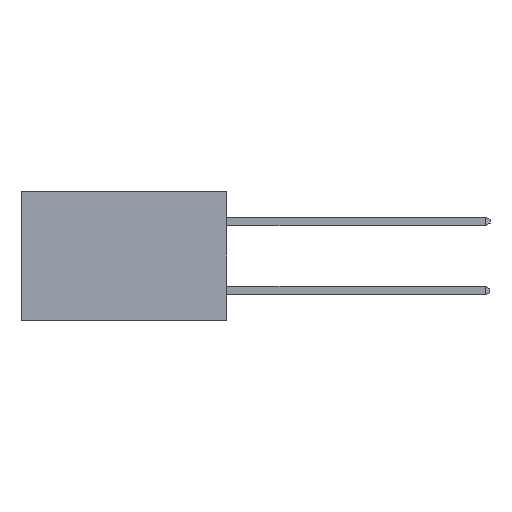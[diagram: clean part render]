
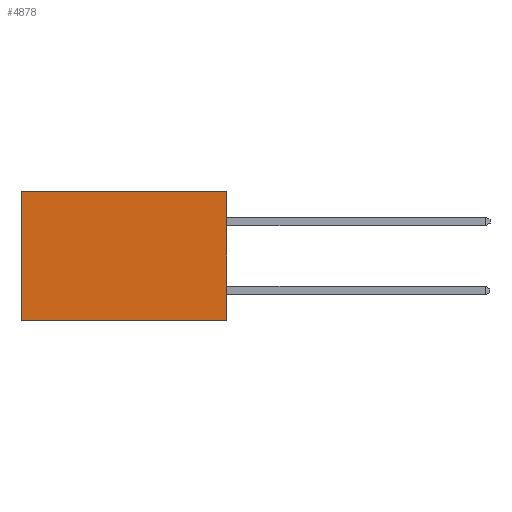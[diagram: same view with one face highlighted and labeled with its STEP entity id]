
A CAD part, left-side view. The second image highlights one B-rep face of the part: STEP entity #4878.
In plain terms, the highlighted planar face has unit normal (-1, 0, 0).
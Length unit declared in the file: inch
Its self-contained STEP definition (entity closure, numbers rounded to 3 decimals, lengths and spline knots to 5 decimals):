
#262 = VERTEX_POINT ( 'NONE', #10888 ) ;
#295 = ORIENTED_EDGE ( 'NONE', *, *, #1447, .F. ) ;
#546 = ORIENTED_EDGE ( 'NONE', *, *, #5599, .F. ) ;
#655 = ORIENTED_EDGE ( 'NONE', *, *, #930, .T. ) ;
#930 = EDGE_CURVE ( 'NONE', #1466, #262, #5313, .T. ) ;
#1001 = LINE ( 'NONE', #2396, #2843 ) ;
#1375 = EDGE_CURVE ( 'NONE', #262, #5024, #5073, .T. ) ;
#1444 = ORIENTED_EDGE ( 'NONE', *, *, #1375, .T. ) ;
#1447 = EDGE_CURVE ( 'NONE', #11264, #5024, #10744, .T. ) ;
#1466 = VERTEX_POINT ( 'NONE', #10134 ) ;
#2111 = DIRECTION ( 'NONE',  ( 0., 1., 0. ) ) ;
#2130 = AXIS2_PLACEMENT_3D ( 'NONE', #4250, #5791, #5788 ) ;
#2308 = DIRECTION ( 'NONE',  ( 0., 0., -1. ) ) ;
#2396 = CARTESIAN_POINT ( 'NONE',  ( 0.277, 0., -0.37 ) ) ;
#2786 = VECTOR ( 'NONE', #10671, 39.37008 ) ;
#2843 = VECTOR ( 'NONE', #2308, 39.37008 ) ;
#3732 = VECTOR ( 'NONE', #2111, 39.37008 ) ;
#4171 = DIRECTION ( 'NONE',  ( 0., 0., -1. ) ) ;
#4250 = CARTESIAN_POINT ( 'NONE',  ( 0.277, 0., -0.37 ) ) ;
#4266 = PLANE ( 'NONE',  #2130 ) ;
#4386 = CARTESIAN_POINT ( 'NONE',  ( 0.277, 0.59, -0.37 ) ) ;
#4878 = ADVANCED_FACE ( 'NONE', ( #5660 ), #4266, .F. ) ;
#5024 = VERTEX_POINT ( 'NONE', #4386 ) ;
#5073 = LINE ( 'NONE', #5086, #7160 ) ;
#5086 = CARTESIAN_POINT ( 'NONE',  ( 0.277, 0.59, -0.37 ) ) ;
#5313 = LINE ( 'NONE', #10968, #2786 ) ;
#5599 = EDGE_CURVE ( 'NONE', #1466, #11264, #1001, .T. ) ;
#5660 = FACE_OUTER_BOUND ( 'NONE', #10294, .T. ) ;
#5788 = DIRECTION ( 'NONE',  ( 0., 0., -1. ) ) ;
#5791 = DIRECTION ( 'NONE',  ( 1., 0., 0. ) ) ;
#7160 = VECTOR ( 'NONE', #4171, 39.37008 ) ;
#10134 = CARTESIAN_POINT ( 'NONE',  ( 0.277, 0., 0. ) ) ;
#10294 = EDGE_LOOP ( 'NONE', ( #1444, #295, #546, #655 ) ) ;
#10394 = CARTESIAN_POINT ( 'NONE',  ( 0.277, 0., -0.37 ) ) ;
#10492 = CARTESIAN_POINT ( 'NONE',  ( 0.277, 0., -0.37 ) ) ;
#10671 = DIRECTION ( 'NONE',  ( 0., 1., 0. ) ) ;
#10744 = LINE ( 'NONE', #10492, #3732 ) ;
#10888 = CARTESIAN_POINT ( 'NONE',  ( 0.277, 0.59, 0. ) ) ;
#10968 = CARTESIAN_POINT ( 'NONE',  ( 0.277, 0., 0. ) ) ;
#11264 = VERTEX_POINT ( 'NONE', #10394 ) ;
